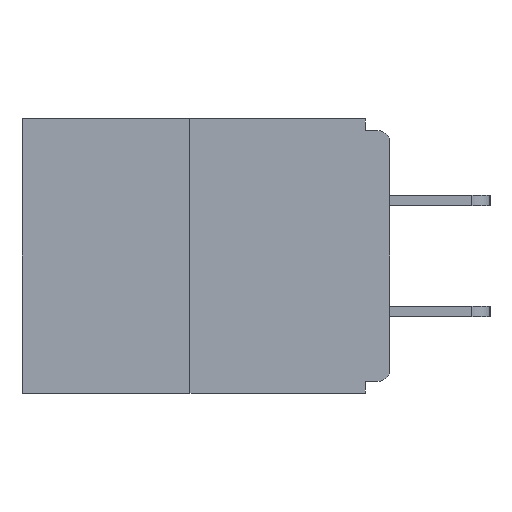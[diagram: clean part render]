
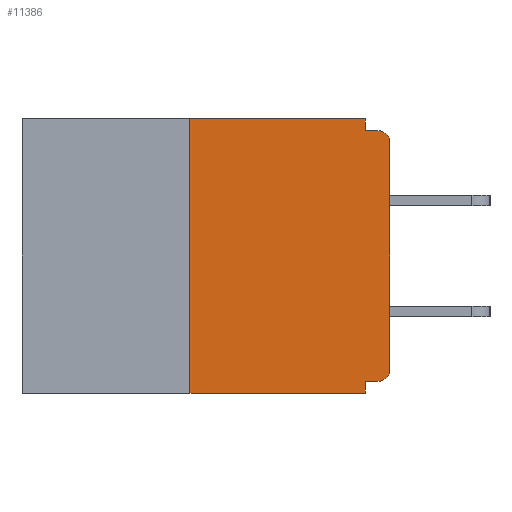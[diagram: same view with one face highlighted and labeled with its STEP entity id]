
A CAD part, left-side view. The second image highlights one B-rep face of the part: STEP entity #11386.
In plain terms, the highlighted planar face has unit normal (-1, 0, 0).
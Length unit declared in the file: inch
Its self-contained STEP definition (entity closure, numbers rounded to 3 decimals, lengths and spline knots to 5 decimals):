
#11 = CARTESIAN_POINT ( 'NONE',  ( 0., 0.031, 0. ) ) ;
#234 = LINE ( 'NONE', #304, #6224 ) ;
#304 = CARTESIAN_POINT ( 'NONE',  ( 0., 0.46, 0. ) ) ;
#485 = VECTOR ( 'NONE', #7888, 39.37008 ) ;
#494 = DIRECTION ( 'NONE',  ( 0., 0., 1. ) ) ;
#705 = CARTESIAN_POINT ( 'NONE',  ( 0., 0.031, -0.328 ) ) ;
#1209 = CARTESIAN_POINT ( 'NONE',  ( 0., 0.25, 0. ) ) ;
#1241 = VERTEX_POINT ( 'NONE', #9211 ) ;
#1315 = CARTESIAN_POINT ( 'NONE',  ( 0., 0.031, -0.343 ) ) ;
#1359 = VERTEX_POINT ( 'NONE', #7431 ) ;
#1436 = CARTESIAN_POINT ( 'NONE',  ( 0., 0.031, -0.015 ) ) ;
#1575 = LINE ( 'NONE', #12390, #3274 ) ;
#1617 = LINE ( 'NONE', #13832, #10507 ) ;
#1661 = ORIENTED_EDGE ( 'NONE', *, *, #7002, .F. ) ;
#1972 = ORIENTED_EDGE ( 'NONE', *, *, #3401, .T. ) ;
#2185 = CARTESIAN_POINT ( 'NONE',  ( 0., 0.25, -0.343 ) ) ;
#2212 = LINE ( 'NONE', #1209, #8277 ) ;
#2399 = DIRECTION ( 'NONE',  ( 0., 0., -1. ) ) ;
#2479 = VERTEX_POINT ( 'NONE', #8912 ) ;
#2606 = ORIENTED_EDGE ( 'NONE', *, *, #8022, .T. ) ;
#2741 = VERTEX_POINT ( 'NONE', #1315 ) ;
#3274 = VECTOR ( 'NONE', #13516, 39.37008 ) ;
#3386 = LINE ( 'NONE', #11, #485 ) ;
#3401 = EDGE_CURVE ( 'NONE', #6769, #8179, #6862, .T. ) ;
#3690 = VERTEX_POINT ( 'NONE', #1436 ) ;
#3777 = EDGE_LOOP ( 'NONE', ( #13390, #7757, #8318, #1661, #8215, #13663, #1972, #2606, #4824, #4238 ) ) ;
#3854 = FACE_OUTER_BOUND ( 'NONE', #3777, .T. ) ;
#4238 = ORIENTED_EDGE ( 'NONE', *, *, #6012, .F. ) ;
#4493 = EDGE_CURVE ( 'NONE', #1359, #1241, #234, .T. ) ;
#4690 = DIRECTION ( 'NONE',  ( 0., -1., 0. ) ) ;
#4768 = LINE ( 'NONE', #6991, #6677 ) ;
#4824 = ORIENTED_EDGE ( 'NONE', *, *, #8278, .F. ) ;
#5125 = EDGE_CURVE ( 'NONE', #2479, #6769, #5337, .T. ) ;
#5337 = CIRCLE ( 'NONE', #13727, 0.015 ) ;
#5497 = DIRECTION ( 'NONE',  ( -1., 0., 0. ) ) ;
#5959 = CARTESIAN_POINT ( 'NONE',  ( 0., 0., -0.03 ) ) ;
#6012 = EDGE_CURVE ( 'NONE', #1241, #3690, #3386, .T. ) ;
#6224 = VECTOR ( 'NONE', #8945, 39.37008 ) ;
#6630 = DIRECTION ( 'NONE',  ( 0., 0., -1. ) ) ;
#6677 = VECTOR ( 'NONE', #9124, 39.37008 ) ;
#6769 = VERTEX_POINT ( 'NONE', #12876 ) ;
#6862 = LINE ( 'NONE', #11188, #11924 ) ;
#6991 = CARTESIAN_POINT ( 'NONE',  ( 0., 0., -0.328 ) ) ;
#7002 = EDGE_CURVE ( 'NONE', #13684, #2741, #1575, .T. ) ;
#7119 = DIRECTION ( 'NONE',  ( 1., 0., 0. ) ) ;
#7431 = CARTESIAN_POINT ( 'NONE',  ( 0., 0.25, 0. ) ) ;
#7614 = CARTESIAN_POINT ( 'NONE',  ( 0., 0.015, -0.03 ) ) ;
#7757 = ORIENTED_EDGE ( 'NONE', *, *, #13957, .F. ) ;
#7888 = DIRECTION ( 'NONE',  ( 0., 0., -1. ) ) ;
#8022 = EDGE_CURVE ( 'NONE', #8179, #12588, #12406, .T. ) ;
#8058 = DIRECTION ( 'NONE',  ( 0., 0., -1. ) ) ;
#8179 = VERTEX_POINT ( 'NONE', #5959 ) ;
#8199 = PLANE ( 'NONE',  #13031 ) ;
#8215 = ORIENTED_EDGE ( 'NONE', *, *, #12205, .F. ) ;
#8277 = VECTOR ( 'NONE', #10123, 39.37008 ) ;
#8278 = EDGE_CURVE ( 'NONE', #3690, #12588, #1617, .T. ) ;
#8318 = ORIENTED_EDGE ( 'NONE', *, *, #13074, .T. ) ;
#8912 = CARTESIAN_POINT ( 'NONE',  ( 0., 0.015, -0.328 ) ) ;
#8945 = DIRECTION ( 'NONE',  ( 0., -1., 0. ) ) ;
#8986 = CARTESIAN_POINT ( 'NONE',  ( 0., 0.015, -0.015 ) ) ;
#9124 = DIRECTION ( 'NONE',  ( 0., 1., 0. ) ) ;
#9211 = CARTESIAN_POINT ( 'NONE',  ( 0., 0.031, 0. ) ) ;
#9521 = DIRECTION ( 'NONE',  ( 0., -1., 0. ) ) ;
#9807 = VERTEX_POINT ( 'NONE', #2185 ) ;
#10123 = DIRECTION ( 'NONE',  ( 0., 0., 1. ) ) ;
#10140 = AXIS2_PLACEMENT_3D ( 'NONE', #7614, #11944, #2399 ) ;
#10507 = VECTOR ( 'NONE', #9521, 39.37008 ) ;
#11089 = LINE ( 'NONE', #12085, #11184 ) ;
#11184 = VECTOR ( 'NONE', #4690, 39.37008 ) ;
#11188 = CARTESIAN_POINT ( 'NONE',  ( 0., 0., 0. ) ) ;
#11386 = ADVANCED_FACE ( 'NONE', ( #3854 ), #8199, .F. ) ;
#11924 = VECTOR ( 'NONE', #494, 39.37008 ) ;
#11944 = DIRECTION ( 'NONE',  ( -1., 0., 0. ) ) ;
#12085 = CARTESIAN_POINT ( 'NONE',  ( 0., 0.46, -0.343 ) ) ;
#12205 = EDGE_CURVE ( 'NONE', #2479, #13684, #4768, .T. ) ;
#12390 = CARTESIAN_POINT ( 'NONE',  ( 0., 0.031, -0.343 ) ) ;
#12406 = CIRCLE ( 'NONE', #10140, 0.015 ) ;
#12583 = CARTESIAN_POINT ( 'NONE',  ( 0., 0.46, 0. ) ) ;
#12588 = VERTEX_POINT ( 'NONE', #8986 ) ;
#12876 = CARTESIAN_POINT ( 'NONE',  ( 0., 0., -0.313 ) ) ;
#13031 = AXIS2_PLACEMENT_3D ( 'NONE', #12583, #7119, #8058 ) ;
#13074 = EDGE_CURVE ( 'NONE', #9807, #2741, #11089, .T. ) ;
#13390 = ORIENTED_EDGE ( 'NONE', *, *, #4493, .F. ) ;
#13516 = DIRECTION ( 'NONE',  ( 0., 0., -1. ) ) ;
#13663 = ORIENTED_EDGE ( 'NONE', *, *, #5125, .T. ) ;
#13684 = VERTEX_POINT ( 'NONE', #705 ) ;
#13727 = AXIS2_PLACEMENT_3D ( 'NONE', #14031, #5497, #6630 ) ;
#13832 = CARTESIAN_POINT ( 'NONE',  ( 0., 0., -0.015 ) ) ;
#13957 = EDGE_CURVE ( 'NONE', #9807, #1359, #2212, .T. ) ;
#14031 = CARTESIAN_POINT ( 'NONE',  ( 0., 0.015, -0.313 ) ) ;
